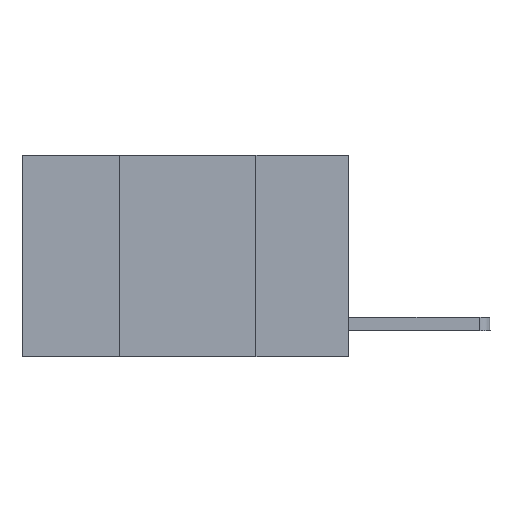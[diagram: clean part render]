
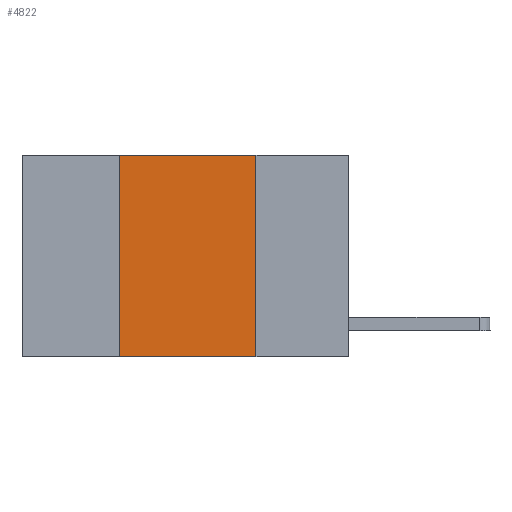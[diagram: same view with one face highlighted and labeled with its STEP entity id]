
A CAD part, left-side view. The second image highlights one B-rep face of the part: STEP entity #4822.
In plain terms, the highlighted planar face has unit normal (-1, 0, 0).
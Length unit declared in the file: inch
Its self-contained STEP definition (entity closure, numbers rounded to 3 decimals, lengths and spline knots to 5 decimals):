
#3 = DIRECTION ( 'NONE',  ( 0., -1., 0. ) ) ;
#93 = CARTESIAN_POINT ( 'NONE',  ( 0., 0.6, -0.37 ) ) ;
#498 = PLANE ( 'NONE',  #1116 ) ;
#944 = CARTESIAN_POINT ( 'NONE',  ( 0., 0.42, 0. ) ) ;
#1116 = AXIS2_PLACEMENT_3D ( 'NONE', #3860, #1141, #8562 ) ;
#1141 = DIRECTION ( 'NONE',  ( 1., 0., 0. ) ) ;
#1575 = CARTESIAN_POINT ( 'NONE',  ( 0., 0.6, 0. ) ) ;
#1844 = FACE_OUTER_BOUND ( 'NONE', #8564, .T. ) ;
#2316 = EDGE_CURVE ( 'NONE', #3231, #5755, #5051, .T. ) ;
#2540 = EDGE_CURVE ( 'NONE', #4295, #7252, #4137, .T. ) ;
#3027 = LINE ( 'NONE', #6990, #4515 ) ;
#3231 = VERTEX_POINT ( 'NONE', #944 ) ;
#3784 = VECTOR ( 'NONE', #3, 39.37008 ) ;
#3860 = CARTESIAN_POINT ( 'NONE',  ( 0., 0.6, 0. ) ) ;
#4137 = LINE ( 'NONE', #93, #3784 ) ;
#4295 = VERTEX_POINT ( 'NONE', #8116 ) ;
#4515 = VECTOR ( 'NONE', #5684, 39.37008 ) ;
#4538 = LINE ( 'NONE', #7184, #6166 ) ;
#4809 = ORIENTED_EDGE ( 'NONE', *, *, #2316, .F. ) ;
#4822 = ADVANCED_FACE ( 'NONE', ( #1844 ), #498, .F. ) ;
#4887 = VECTOR ( 'NONE', #7694, 39.37008 ) ;
#5051 = LINE ( 'NONE', #1575, #4887 ) ;
#5684 = DIRECTION ( 'NONE',  ( 0., 0., 1. ) ) ;
#5755 = VERTEX_POINT ( 'NONE', #6781 ) ;
#6166 = VECTOR ( 'NONE', #8390, 39.37008 ) ;
#6732 = EDGE_CURVE ( 'NONE', #5755, #7252, #4538, .T. ) ;
#6779 = ORIENTED_EDGE ( 'NONE', *, *, #6732, .F. ) ;
#6781 = CARTESIAN_POINT ( 'NONE',  ( 0., 0.17, 0. ) ) ;
#6990 = CARTESIAN_POINT ( 'NONE',  ( 0., 0.42, 0. ) ) ;
#7184 = CARTESIAN_POINT ( 'NONE',  ( 0., 0.17, 0. ) ) ;
#7252 = VERTEX_POINT ( 'NONE', #7636 ) ;
#7275 = ORIENTED_EDGE ( 'NONE', *, *, #7561, .F. ) ;
#7490 = ORIENTED_EDGE ( 'NONE', *, *, #2540, .T. ) ;
#7561 = EDGE_CURVE ( 'NONE', #4295, #3231, #3027, .T. ) ;
#7636 = CARTESIAN_POINT ( 'NONE',  ( 0., 0.17, -0.37 ) ) ;
#7694 = DIRECTION ( 'NONE',  ( 0., -1., 0. ) ) ;
#8116 = CARTESIAN_POINT ( 'NONE',  ( 0., 0.42, -0.37 ) ) ;
#8390 = DIRECTION ( 'NONE',  ( 0., 0., -1. ) ) ;
#8562 = DIRECTION ( 'NONE',  ( 0., 0., -1. ) ) ;
#8564 = EDGE_LOOP ( 'NONE', ( #6779, #4809, #7275, #7490 ) ) ;
